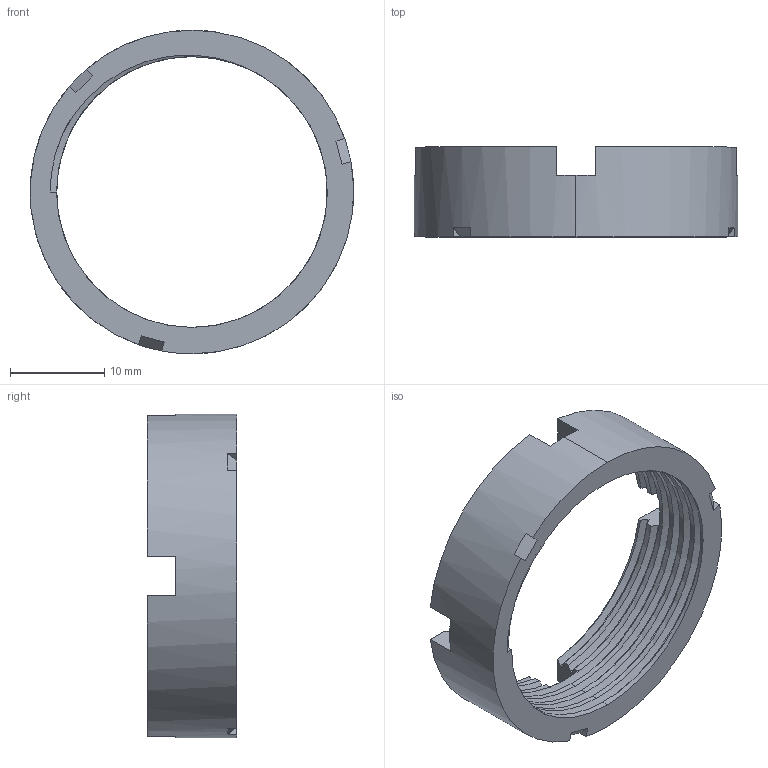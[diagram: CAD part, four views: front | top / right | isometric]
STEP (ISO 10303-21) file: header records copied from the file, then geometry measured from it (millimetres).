
FILE_DESCRIPTION (( 'STEP AP214' ), '1' );
FILE_NAME ('User Library-Telescopic Stock_5310-917-1154.STEP', '2013-05-23T12:58:18', ( 'Asher' ), ( '' ), 'SwSTEP 2.0', 'SolidWorks 2013', '' );
FILE_SCHEMA (( 'AUTOMOTIVE_DESIGN' ));
Length unit declared in the file: millimetre
Products named in the file (1): User Library-Telescopic Stock_5310-917-1154
Bounding box: 34.4 x 9.55 x 34.42 mm (x, y, z)
Volume: 2306.8 mm3; surface area: 2798.6 mm2
Topology: 1 solids, 1 shells, 79 faces, 234 edges, 156 vertices
Faces by surface type: cylinder 36, plane 27, bspline 16
Entity records: 4269 total; most frequent: CARTESIAN_POINT 2434, ORIENTED_EDGE 468, DIRECTION 280, EDGE_CURVE 234, VERTEX_POINT 156, LINE 102, VECTOR 102, AXIS2_PLACEMENT_3D 89
